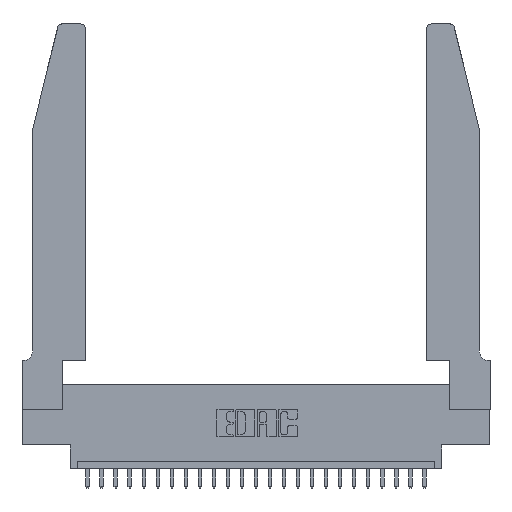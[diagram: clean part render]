
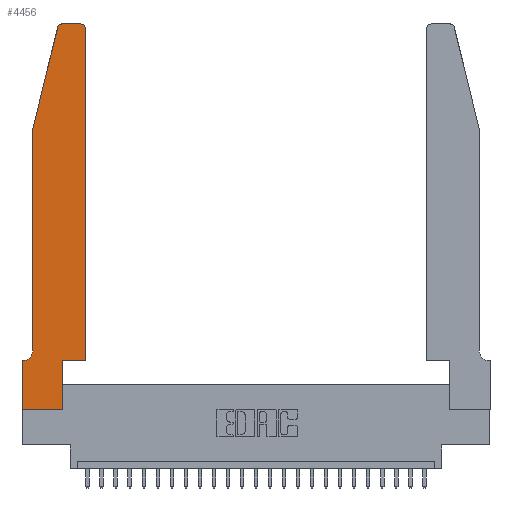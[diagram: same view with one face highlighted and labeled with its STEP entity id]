
A CAD part, top view. The second image highlights one B-rep face of the part: STEP entity #4456.
In plain terms, the highlighted planar face has unit normal (0, 0, 1).
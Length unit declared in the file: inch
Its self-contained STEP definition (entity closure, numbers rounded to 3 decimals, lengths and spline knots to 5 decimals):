
#62 = CIRCLE ( 'NONE', #23930, 0.03 ) ;
#151 = LINE ( 'NONE', #18490, #1755 ) ;
#1281 = LINE ( 'NONE', #3951, #3463 ) ;
#1418 = VERTEX_POINT ( 'NONE', #3474 ) ;
#1436 = CARTESIAN_POINT ( 'NONE',  ( 0.0755, 2., 0.37 ) ) ;
#1455 = VECTOR ( 'NONE', #18677, 39.37008 ) ;
#1464 = EDGE_CURVE ( 'NONE', #14832, #13325, #20753, .T. ) ;
#1543 = LINE ( 'NONE', #8071, #11605 ) ;
#1546 = ORIENTED_EDGE ( 'NONE', *, *, #4633, .T. ) ;
#1755 = VECTOR ( 'NONE', #2407, 39.37008 ) ;
#1948 = LINE ( 'NONE', #14807, #5133 ) ;
#2407 = DIRECTION ( 'NONE',  ( 1., 0., 0. ) ) ;
#2495 = VERTEX_POINT ( 'NONE', #6441 ) ;
#2760 = EDGE_LOOP ( 'NONE', ( #25253, #12136, #20369, #24480, #1546, #11822, #22376, #18889, #25328, #12795, #3451, #13088 ) ) ;
#3124 = VERTEX_POINT ( 'NONE', #22323 ) ;
#3154 = DIRECTION ( 'NONE',  ( 1., 0., 0. ) ) ;
#3338 = CIRCLE ( 'NONE', #9131, 0.07 ) ;
#3451 = ORIENTED_EDGE ( 'NONE', *, *, #3775, .T. ) ;
#3463 = VECTOR ( 'NONE', #5408, 39.37008 ) ;
#3474 = CARTESIAN_POINT ( 'NONE',  ( 0.4505, 0.35, 0.37 ) ) ;
#3736 = VECTOR ( 'NONE', #19913, 39.37008 ) ;
#3775 = EDGE_CURVE ( 'NONE', #1418, #17927, #7776, .T. ) ;
#3951 = CARTESIAN_POINT ( 'NONE',  ( 0.2865, 0.35, 0.37 ) ) ;
#4161 = CARTESIAN_POINT ( 'NONE',  ( 0.0755, 0.42, 0.37 ) ) ;
#4170 = EDGE_CURVE ( 'NONE', #23932, #1418, #151, .T. ) ;
#4431 = CARTESIAN_POINT ( 'NONE',  ( 0.2865, 0.35, 0.37 ) ) ;
#4456 = ADVANCED_FACE ( 'NONE', ( #7726 ), #14037, .T. ) ;
#4633 = EDGE_CURVE ( 'NONE', #19705, #2495, #3338, .T. ) ;
#4659 = VERTEX_POINT ( 'NONE', #18826 ) ;
#4827 = VERTEX_POINT ( 'NONE', #10925 ) ;
#5133 = VECTOR ( 'NONE', #21001, 39.37008 ) ;
#5281 = DIRECTION ( 'NONE',  ( 1., 0., 0. ) ) ;
#5408 = DIRECTION ( 'NONE',  ( 0., 1., 0. ) ) ;
#5531 = EDGE_CURVE ( 'NONE', #4827, #14832, #22363, .T. ) ;
#5978 = CARTESIAN_POINT ( 'NONE',  ( 0.0755, 2., 0.37 ) ) ;
#6441 = CARTESIAN_POINT ( 'NONE',  ( 0.0055, 0.35, 0.37 ) ) ;
#6706 = EDGE_CURVE ( 'NONE', #4659, #24799, #1948, .T. ) ;
#6738 = CARTESIAN_POINT ( 'NONE',  ( 0.25487, 2.72718, 0.37 ) ) ;
#6953 = LINE ( 'NONE', #22329, #11920 ) ;
#7068 = AXIS2_PLACEMENT_3D ( 'NONE', #15078, #11247, #5281 ) ;
#7473 = EDGE_CURVE ( 'NONE', #24799, #23932, #1281, .T. ) ;
#7726 = FACE_OUTER_BOUND ( 'NONE', #2760, .T. ) ;
#7776 = LINE ( 'NONE', #25978, #15866 ) ;
#8071 = CARTESIAN_POINT ( 'NONE',  ( 0., 0., 0.37 ) ) ;
#9131 = AXIS2_PLACEMENT_3D ( 'NONE', #10802, #20847, #10887 ) ;
#9315 = CARTESIAN_POINT ( 'NONE',  ( 0.4205, 2.72, 0.37 ) ) ;
#9934 = LINE ( 'NONE', #20597, #1455 ) ;
#10482 = CARTESIAN_POINT ( 'NONE',  ( 0.284, 2.75, 0.37 ) ) ;
#10802 = CARTESIAN_POINT ( 'NONE',  ( 0.0055, 0.42, 0.37 ) ) ;
#10887 = DIRECTION ( 'NONE',  ( -1., 0., 0. ) ) ;
#10925 = CARTESIAN_POINT ( 'NONE',  ( 0.4205, 2.75, 0.37 ) ) ;
#11247 = DIRECTION ( 'NONE',  ( 0., 0., 1. ) ) ;
#11605 = VECTOR ( 'NONE', #22204, 39.37008 ) ;
#11822 = ORIENTED_EDGE ( 'NONE', *, *, #13137, .T. ) ;
#11920 = VECTOR ( 'NONE', #24458, 39.37008 ) ;
#12136 = ORIENTED_EDGE ( 'NONE', *, *, #1464, .T. ) ;
#12795 = ORIENTED_EDGE ( 'NONE', *, *, #4170, .T. ) ;
#13088 = ORIENTED_EDGE ( 'NONE', *, *, #15674, .T. ) ;
#13137 = EDGE_CURVE ( 'NONE', #2495, #3124, #9934, .T. ) ;
#13325 = VERTEX_POINT ( 'NONE', #6738 ) ;
#13340 = DIRECTION ( 'NONE',  ( 1., 0., 0. ) ) ;
#13475 = CARTESIAN_POINT ( 'NONE',  ( 0.2865, 0., 0.37 ) ) ;
#13639 = VERTEX_POINT ( 'NONE', #1436 ) ;
#14037 = PLANE ( 'NONE',  #17285 ) ;
#14807 = CARTESIAN_POINT ( 'NONE',  ( 0., 0., 0.37 ) ) ;
#14832 = VERTEX_POINT ( 'NONE', #10482 ) ;
#15078 = CARTESIAN_POINT ( 'NONE',  ( 0.284, 2.72, 0.37 ) ) ;
#15674 = EDGE_CURVE ( 'NONE', #17927, #4827, #62, .T. ) ;
#15866 = VECTOR ( 'NONE', #19970, 39.37008 ) ;
#16401 = CARTESIAN_POINT ( 'NONE',  ( 0.2605, 2.75, 0.37 ) ) ;
#17285 = AXIS2_PLACEMENT_3D ( 'NONE', #18599, #21239, #3154 ) ;
#17927 = VERTEX_POINT ( 'NONE', #18963 ) ;
#18490 = CARTESIAN_POINT ( 'NONE',  ( 0.4505, 0.35, 0.37 ) ) ;
#18599 = CARTESIAN_POINT ( 'NONE',  ( 0., 0.35, 0.37 ) ) ;
#18617 = EDGE_CURVE ( 'NONE', #13325, #13639, #6953, .T. ) ;
#18677 = DIRECTION ( 'NONE',  ( -1., 0., 0. ) ) ;
#18826 = CARTESIAN_POINT ( 'NONE',  ( 0., 0., 0.37 ) ) ;
#18889 = ORIENTED_EDGE ( 'NONE', *, *, #6706, .T. ) ;
#18933 = VECTOR ( 'NONE', #22209, 39.37008 ) ;
#18963 = CARTESIAN_POINT ( 'NONE',  ( 0.4505, 2.72, 0.37 ) ) ;
#19024 = EDGE_CURVE ( 'NONE', #3124, #4659, #1543, .T. ) ;
#19705 = VERTEX_POINT ( 'NONE', #4161 ) ;
#19913 = DIRECTION ( 'NONE',  ( 0., -1., 0. ) ) ;
#19970 = DIRECTION ( 'NONE',  ( 0., 1., 0. ) ) ;
#20369 = ORIENTED_EDGE ( 'NONE', *, *, #18617, .T. ) ;
#20597 = CARTESIAN_POINT ( 'NONE',  ( 0.0755, 0.35, 0.37 ) ) ;
#20753 = CIRCLE ( 'NONE', #7068, 0.03 ) ;
#20847 = DIRECTION ( 'NONE',  ( 0., 0., -1. ) ) ;
#21001 = DIRECTION ( 'NONE',  ( 1., 0., 0. ) ) ;
#21239 = DIRECTION ( 'NONE',  ( 0., 0., 1. ) ) ;
#22204 = DIRECTION ( 'NONE',  ( 0., -1., 0. ) ) ;
#22209 = DIRECTION ( 'NONE',  ( -1., 0., 0. ) ) ;
#22323 = CARTESIAN_POINT ( 'NONE',  ( 0., 0.35, 0.37 ) ) ;
#22329 = CARTESIAN_POINT ( 'NONE',  ( 0.0755, 2., 0.37 ) ) ;
#22363 = LINE ( 'NONE', #16401, #18933 ) ;
#22376 = ORIENTED_EDGE ( 'NONE', *, *, #19024, .T. ) ;
#22536 = LINE ( 'NONE', #5978, #3736 ) ;
#23279 = DIRECTION ( 'NONE',  ( 0., 0., 1. ) ) ;
#23930 = AXIS2_PLACEMENT_3D ( 'NONE', #9315, #23279, #13340 ) ;
#23932 = VERTEX_POINT ( 'NONE', #4431 ) ;
#24417 = EDGE_CURVE ( 'NONE', #13639, #19705, #22536, .T. ) ;
#24458 = DIRECTION ( 'NONE',  ( -0.239, -0.971, 0. ) ) ;
#24480 = ORIENTED_EDGE ( 'NONE', *, *, #24417, .T. ) ;
#24799 = VERTEX_POINT ( 'NONE', #13475 ) ;
#25253 = ORIENTED_EDGE ( 'NONE', *, *, #5531, .T. ) ;
#25328 = ORIENTED_EDGE ( 'NONE', *, *, #7473, .T. ) ;
#25978 = CARTESIAN_POINT ( 'NONE',  ( 0.4505, 0.35, 0.37 ) ) ;
